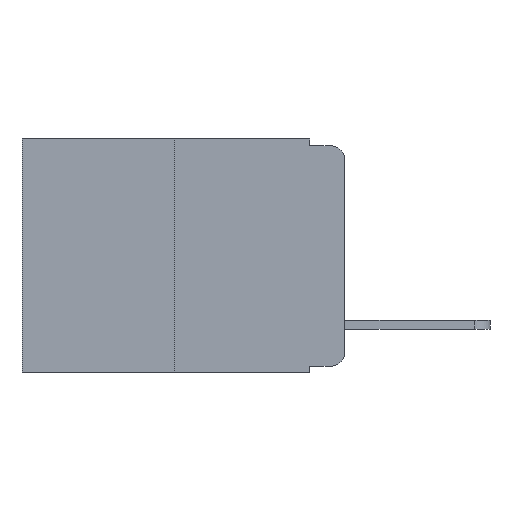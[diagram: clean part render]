
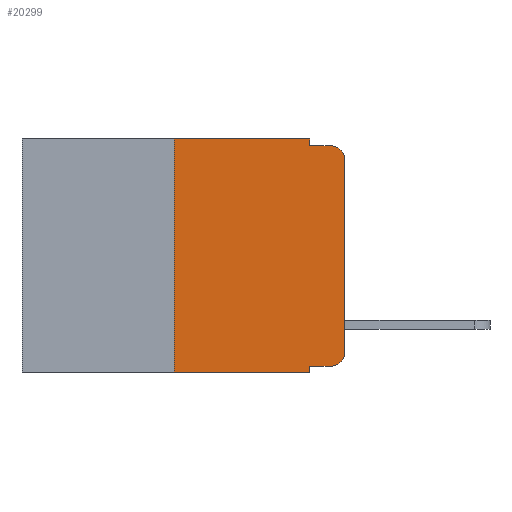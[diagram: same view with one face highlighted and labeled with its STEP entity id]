
A CAD part, left-side view. The second image highlights one B-rep face of the part: STEP entity #20299.
In plain terms, the highlighted planar face has unit normal (-1, 0, 0).
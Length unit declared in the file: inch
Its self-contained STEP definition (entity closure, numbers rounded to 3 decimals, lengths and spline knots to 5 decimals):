
#79 = CARTESIAN_POINT ( 'NONE',  ( 0., 0.051, -0.01 ) ) ;
#563 = CARTESIAN_POINT ( 'NONE',  ( 0., 0.473, 0. ) ) ;
#964 = ORIENTED_EDGE ( 'NONE', *, *, #21719, .T. ) ;
#1472 = DIRECTION ( 'NONE',  ( 0., -1., 0. ) ) ;
#1616 = ORIENTED_EDGE ( 'NONE', *, *, #18720, .F. ) ;
#1617 = VERTEX_POINT ( 'NONE', #5025 ) ;
#1633 = CARTESIAN_POINT ( 'NONE',  ( 0., 0.051, -0.333 ) ) ;
#1954 = LINE ( 'NONE', #2252, #20391 ) ;
#2000 = VERTEX_POINT ( 'NONE', #16434 ) ;
#2252 = CARTESIAN_POINT ( 'NONE',  ( 0., 0.473, -0.343 ) ) ;
#2683 = DIRECTION ( 'NONE',  ( 0., 0., -1. ) ) ;
#3245 = VERTEX_POINT ( 'NONE', #16252 ) ;
#4114 = VERTEX_POINT ( 'NONE', #12639 ) ;
#4224 = DIRECTION ( 'NONE',  ( -1., 0., 0. ) ) ;
#4742 = VERTEX_POINT ( 'NONE', #9609 ) ;
#5025 = CARTESIAN_POINT ( 'NONE',  ( 0., 0.02, -0.333 ) ) ;
#5083 = VERTEX_POINT ( 'NONE', #1633 ) ;
#5147 = DIRECTION ( 'NONE',  ( -1., 0., 0. ) ) ;
#5340 = DIRECTION ( 'NONE',  ( 0., 0., -1. ) ) ;
#5698 = DIRECTION ( 'NONE',  ( 0., -1., 0. ) ) ;
#5954 = VERTEX_POINT ( 'NONE', #21576 ) ;
#6314 = VECTOR ( 'NONE', #19312, 39.37008 ) ;
#6559 = VECTOR ( 'NONE', #5340, 39.37008 ) ;
#6827 = VERTEX_POINT ( 'NONE', #20580 ) ;
#6863 = CARTESIAN_POINT ( 'NONE',  ( 0., 0.051, 0. ) ) ;
#6942 = LINE ( 'NONE', #12217, #15431 ) ;
#7606 = CARTESIAN_POINT ( 'NONE',  ( 0., 0.051, -0.01 ) ) ;
#7648 = LINE ( 'NONE', #6863, #17282 ) ;
#7680 = LINE ( 'NONE', #16503, #20091 ) ;
#7705 = ORIENTED_EDGE ( 'NONE', *, *, #7921, .T. ) ;
#7921 = EDGE_CURVE ( 'NONE', #6827, #14518, #1954, .T. ) ;
#8221 = ORIENTED_EDGE ( 'NONE', *, *, #18812, .F. ) ;
#9609 = CARTESIAN_POINT ( 'NONE',  ( 0., 0.051, 0. ) ) ;
#9807 = VECTOR ( 'NONE', #13126, 39.37008 ) ;
#9977 = PLANE ( 'NONE',  #12830 ) ;
#10730 = CARTESIAN_POINT ( 'NONE',  ( 0., 0.473, 0. ) ) ;
#10895 = ORIENTED_EDGE ( 'NONE', *, *, #20520, .T. ) ;
#11366 = LINE ( 'NONE', #19395, #6559 ) ;
#11516 = EDGE_LOOP ( 'NONE', ( #964, #10895, #15658, #1616, #16229, #20651, #7705, #8221, #13044, #17865 ) ) ;
#12217 = CARTESIAN_POINT ( 'NONE',  ( 0., 0.25, 0. ) ) ;
#12394 = AXIS2_PLACEMENT_3D ( 'NONE', #15922, #5147, #17703 ) ;
#12537 = LINE ( 'NONE', #10730, #21205 ) ;
#12639 = CARTESIAN_POINT ( 'NONE',  ( 0., 0., -0.03 ) ) ;
#12649 = CARTESIAN_POINT ( 'NONE',  ( 0., 0.051, -0.343 ) ) ;
#12830 = AXIS2_PLACEMENT_3D ( 'NONE', #563, #13505, #2683 ) ;
#13044 = ORIENTED_EDGE ( 'NONE', *, *, #21923, .T. ) ;
#13126 = DIRECTION ( 'NONE',  ( 0., -1., 0. ) ) ;
#13505 = DIRECTION ( 'NONE',  ( 1., 0., 0. ) ) ;
#14518 = VERTEX_POINT ( 'NONE', #12649 ) ;
#14620 = DIRECTION ( 'NONE',  ( 0., -1., 0. ) ) ;
#14987 = CARTESIAN_POINT ( 'NONE',  ( 0., 0.02, -0.313 ) ) ;
#15431 = VECTOR ( 'NONE', #15873, 39.37008 ) ;
#15658 = ORIENTED_EDGE ( 'NONE', *, *, #19682, .F. ) ;
#15755 = AXIS2_PLACEMENT_3D ( 'NONE', #14987, #4224, #16834 ) ;
#15871 = DIRECTION ( 'NONE',  ( 0., 0., -1. ) ) ;
#15873 = DIRECTION ( 'NONE',  ( 0., 0., 1. ) ) ;
#15922 = CARTESIAN_POINT ( 'NONE',  ( 0., 0.02, -0.03 ) ) ;
#16229 = ORIENTED_EDGE ( 'NONE', *, *, #21143, .F. ) ;
#16252 = CARTESIAN_POINT ( 'NONE',  ( 0., 0., -0.313 ) ) ;
#16434 = CARTESIAN_POINT ( 'NONE',  ( 0., 0.02, -0.01 ) ) ;
#16503 = CARTESIAN_POINT ( 'NONE',  ( 0., 0.051, -0.333 ) ) ;
#16834 = DIRECTION ( 'NONE',  ( 0., 0., -1. ) ) ;
#17282 = VECTOR ( 'NONE', #15871, 39.37008 ) ;
#17703 = DIRECTION ( 'NONE',  ( 0., 0., -1. ) ) ;
#17727 = CARTESIAN_POINT ( 'NONE',  ( 0., 0., 0. ) ) ;
#17865 = ORIENTED_EDGE ( 'NONE', *, *, #20163, .T. ) ;
#18720 = EDGE_CURVE ( 'NONE', #4742, #22021, #7648, .T. ) ;
#18812 = EDGE_CURVE ( 'NONE', #5083, #14518, #11366, .T. ) ;
#19139 = CIRCLE ( 'NONE', #12394, 0.02 ) ;
#19312 = DIRECTION ( 'NONE',  ( 0., 0., 1. ) ) ;
#19395 = CARTESIAN_POINT ( 'NONE',  ( 0., 0.051, 0. ) ) ;
#19682 = EDGE_CURVE ( 'NONE', #22021, #2000, #22976, .T. ) ;
#19860 = EDGE_CURVE ( 'NONE', #6827, #5954, #6942, .T. ) ;
#20091 = VECTOR ( 'NONE', #5698, 39.37008 ) ;
#20163 = EDGE_CURVE ( 'NONE', #1617, #3245, #20453, .T. ) ;
#20299 = ADVANCED_FACE ( 'NONE', ( #22269 ), #9977, .F. ) ;
#20367 = LINE ( 'NONE', #17727, #6314 ) ;
#20391 = VECTOR ( 'NONE', #14620, 39.37008 ) ;
#20453 = CIRCLE ( 'NONE', #15755, 0.02 ) ;
#20520 = EDGE_CURVE ( 'NONE', #4114, #2000, #19139, .T. ) ;
#20580 = CARTESIAN_POINT ( 'NONE',  ( 0., 0.25, -0.343 ) ) ;
#20651 = ORIENTED_EDGE ( 'NONE', *, *, #19860, .F. ) ;
#21143 = EDGE_CURVE ( 'NONE', #5954, #4742, #12537, .T. ) ;
#21205 = VECTOR ( 'NONE', #1472, 39.37008 ) ;
#21576 = CARTESIAN_POINT ( 'NONE',  ( 0., 0.25, 0. ) ) ;
#21719 = EDGE_CURVE ( 'NONE', #3245, #4114, #20367, .T. ) ;
#21923 = EDGE_CURVE ( 'NONE', #5083, #1617, #7680, .T. ) ;
#22021 = VERTEX_POINT ( 'NONE', #7606 ) ;
#22269 = FACE_OUTER_BOUND ( 'NONE', #11516, .T. ) ;
#22976 = LINE ( 'NONE', #79, #9807 ) ;
